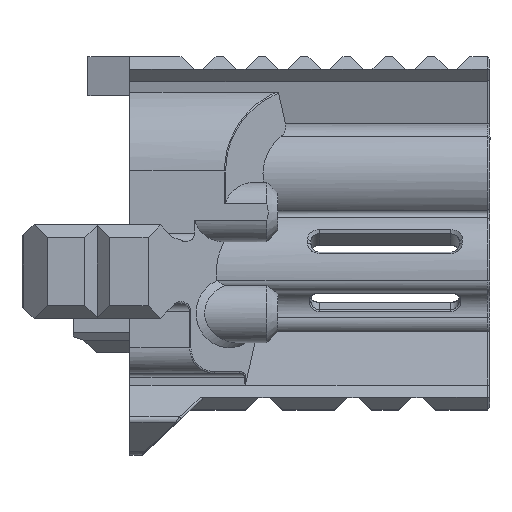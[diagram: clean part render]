
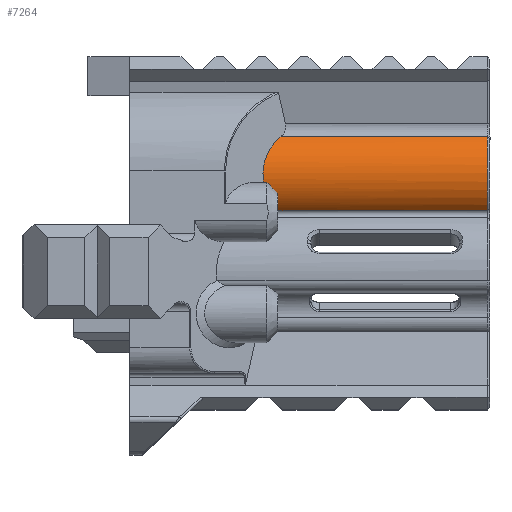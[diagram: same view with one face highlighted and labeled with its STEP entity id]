
A CAD part, top view. The second image highlights one B-rep face of the part: STEP entity #7264.
In plain terms, the highlighted cylindrical face has radius 11.5 mm (diameter 23 mm), a partial arc.
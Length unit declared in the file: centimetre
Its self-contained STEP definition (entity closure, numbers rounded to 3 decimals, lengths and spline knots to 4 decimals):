
#611=LINE($,#12656,#1227);
#612=LINE($,#12723,#1228);
#716=LINE($,#13795,#1332);
#1227=VECTOR($,#9104,4.8783);
#1228=VECTOR($,#9107,0.0705);
#1332=VECTOR($,#9395,5.1159);
#1680=CYLINDRICAL_SURFACE($,#7901,1.15);
#1940=FACE_OUTER_BOUND($,#2407,.T.);
#2407=EDGE_LOOP($,(#6099,#6100,#6101,#6102,#6103,#6104));
#2634=B_SPLINE_CURVE_WITH_KNOTS($,3,(#10282,#10283,#10284,#10285,#10286,
#10287,#10288,#10289,#10290,#10291,#10292,#10293),.UNSPECIFIED.,.F.,.F.,
(4,2,2,2,2,4),(1.7851,1.9083,2.1072,2.3061,
2.5049,2.5782),.UNSPECIFIED.);
#2840=ELLIPSE($,#7806,1.6263,1.15);
#3029=CIRCLE($,#7765,1.15);
#3126=VERTEX_POINT($,#10176);
#3150=VERTEX_POINT($,#10274);
#3151=VERTEX_POINT($,#10281);
#3515=VERTEX_POINT($,#12284);
#3550=VERTEX_POINT($,#12571);
#3551=VERTEX_POINT($,#12573);
#3832=EDGE_CURVE($,#3150,#3151,#2634,.T.);
#4300=EDGE_CURVE($,#3515,#3126,#3029,.T.);
#4372=EDGE_CURVE($,#3551,#3550,#2840,.T.);
#4375=EDGE_CURVE($,#3515,#3551,#611,.T.);
#4378=EDGE_CURVE($,#3151,#3550,#612,.T.);
#4550=EDGE_CURVE($,#3150,#3126,#716,.T.);
#6099=ORIENTED_EDGE($,*,*,#3832,.F.);
#6100=ORIENTED_EDGE($,*,*,#4550,.T.);
#6101=ORIENTED_EDGE($,*,*,#4300,.F.);
#6102=ORIENTED_EDGE($,*,*,#4375,.T.);
#6103=ORIENTED_EDGE($,*,*,#4372,.T.);
#6104=ORIENTED_EDGE($,*,*,#4378,.F.);
#7264=ADVANCED_FACE($,(#1940),#1680,.T.);
#7765=AXIS2_PLACEMENT_3D($,#12288,#8959,#8960);
#7806=AXIS2_PLACEMENT_3D($,#12574,#9098,#9099);
#7901=AXIS2_PLACEMENT_3D($,#13794,#9393,#9394);
#8959=DIRECTION('center_axis',(1.,0.,0.));
#8960=DIRECTION('ref_axis',(0.,0.,1.));
#9098=DIRECTION('center_axis',(0.707,0.,
0.707));
#9099=DIRECTION('ref_axis',(0.707,0.,-0.707));
#9104=DIRECTION($,(-1.,0.,0.));
#9107=DIRECTION($,(-1.,0.,0.));
#9393=DIRECTION('center_axis',(-1.,0.,0.));
#9394=DIRECTION('ref_axis',(0.,-1.,0.));
#9395=DIRECTION($,(1.,0.,0.));
#10176=CARTESIAN_POINT('',(9.619,3.7993,0.8314));
#10274=CARTESIAN_POINT('',(4.5032,3.7993,0.8314));
#10281=CARTESIAN_POINT('',(4.4092,4.4223,1.1934));
#10282=CARTESIAN_POINT('Ctrl Pts',(4.5032,3.7993,0.8314));
#10283=CARTESIAN_POINT('Ctrl Pts',(4.5282,3.8227,0.8577));
#10284=CARTESIAN_POINT('Ctrl Pts',(4.5521,3.8487,0.8846));
#10285=CARTESIAN_POINT('Ctrl Pts',(4.6041,3.9228,0.9534));
#10286=CARTESIAN_POINT('Ctrl Pts',(4.6249,3.9752,0.9947));
#10287=CARTESIAN_POINT('Ctrl Pts',(4.6249,4.0862,1.0672));
#10288=CARTESIAN_POINT('Ctrl Pts',(4.6041,4.1451,1.0985));
#10289=CARTESIAN_POINT('Ctrl Pts',(4.5399,4.2597,1.1482));
#10290=CARTESIAN_POINT('Ctrl Pts',(4.4975,4.3159,1.1668));
#10291=CARTESIAN_POINT('Ctrl Pts',(4.4413,4.3847,1.185));
#10292=CARTESIAN_POINT('Ctrl Pts',(4.4255,4.4035,1.1894));
#10293=CARTESIAN_POINT('Ctrl Pts',(4.4092,4.4223,1.1934));
#12284=CARTESIAN_POINT('',(9.619,5.5535,0.7914));
#12288=CARTESIAN_POINT('Origin',(9.619,4.6595,0.0681));
#12571=CARTESIAN_POINT('',(4.3387,4.4223,1.1934));
#12573=CARTESIAN_POINT('',(4.7407,5.5535,0.7914));
#12574=CARTESIAN_POINT('Origin',(5.464,4.6595,0.0681));
#12656=CARTESIAN_POINT($,(4.579,5.5535,0.7914));
#12723=CARTESIAN_POINT($,(3.6678,4.4223,1.1934));
#13794=CARTESIAN_POINT('Origin',(4.579,4.6595,0.0681));
#13795=CARTESIAN_POINT($,(4.579,3.7993,0.8314));
